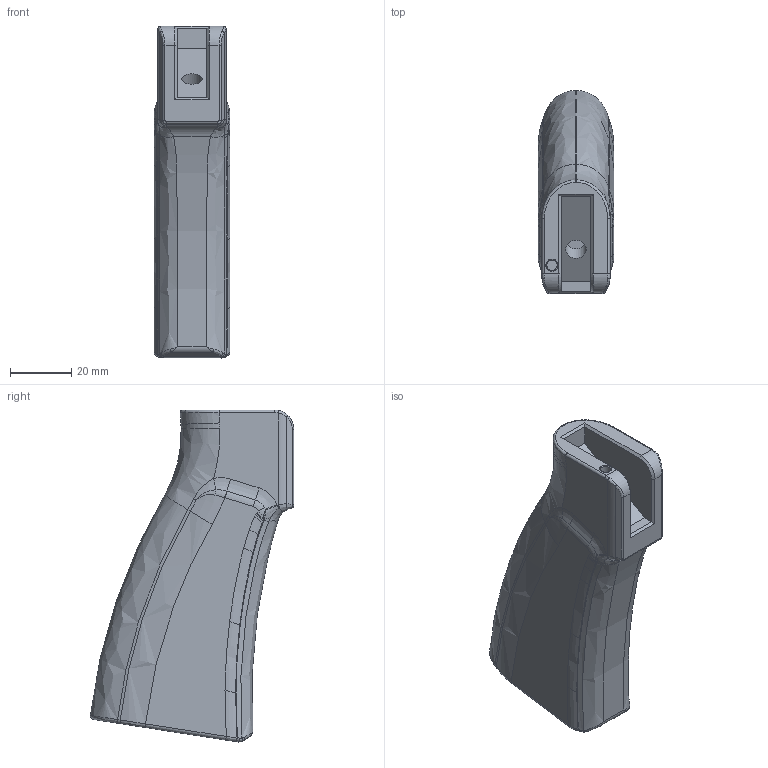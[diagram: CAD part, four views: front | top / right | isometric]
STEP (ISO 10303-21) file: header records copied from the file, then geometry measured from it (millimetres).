
FILE_DESCRIPTION(/* description */ (''),/* implementation_level */ '2;1');
FILE_NAME(/* name */ 'Standard.step',/* time_stamp */ '2021-07-06T20:44:49-04:00',/* author */ (''),/* organization */ (''),/* preprocessor_version */ 'ST-DEVELOPER v18.1',/* originating_system */ 'Autodesk Translation Framework v10.9.0.1377',/* authorisation */ '');
FILE_SCHEMA (('AUTOMOTIVE_DESIGN { 1 0 10303 214 3 1 1 }'));
Length unit declared in the file: millimetre
Products named in the file (1): Standard
Bounding box: 24.83 x 66.65 x 108.78 mm (x, y, z)
Volume: 57204.2 mm3; surface area: 23305.1 mm2
Topology: 1 solids, 1 shells, 274 faces, 647 edges, 364 vertices
Faces by surface type: bspline 140, cylinder 58, plane 36, torus 35, cone 5
Full cylindrical faces by diameter (mm): 3.4 x1, 6.8 x1, 11.05 x1
Entity records: 12278 total; most frequent: CARTESIAN_POINT 6850, ORIENTED_EDGE 1258, DIRECTION 892, EDGE_CURVE 629, AXIS2_PLACEMENT_3D 382, VERTEX_POINT 364, EDGE_LOOP 283, FACE_OUTER_BOUND 274
